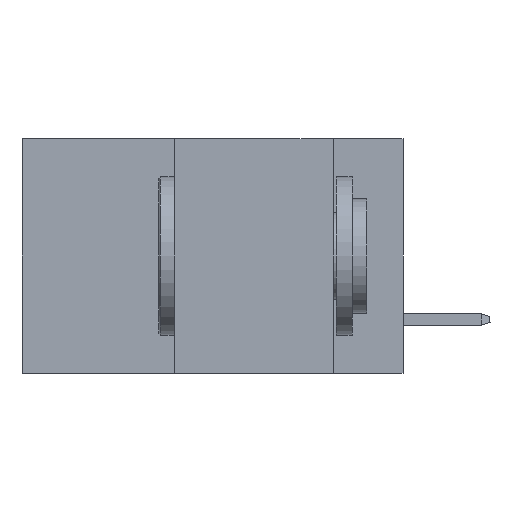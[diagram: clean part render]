
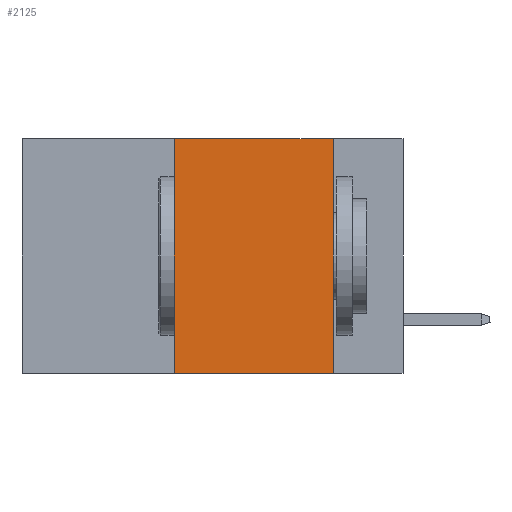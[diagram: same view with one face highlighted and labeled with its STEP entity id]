
A CAD part, left-side view. The second image highlights one B-rep face of the part: STEP entity #2125.
In plain terms, the highlighted planar face has unit normal (-1, 0, 0).
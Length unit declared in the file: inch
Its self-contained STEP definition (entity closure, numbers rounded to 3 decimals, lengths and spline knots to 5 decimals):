
#543 = VECTOR ( 'NONE', #2088, 39.37008 ) ;
#1757 = DIRECTION ( 'NONE',  ( 0., 0., -1. ) ) ;
#2088 = DIRECTION ( 'NONE',  ( 0., -1., 0. ) ) ;
#2125 = ADVANCED_FACE ( 'NONE', ( #6250 ), #36952, .F. ) ;
#2685 = CARTESIAN_POINT ( 'NONE',  ( 0., 0.36, -0.37 ) ) ;
#3008 = ORIENTED_EDGE ( 'NONE', *, *, #6449, .F. ) ;
#3105 = VECTOR ( 'NONE', #20566, 39.37008 ) ;
#5437 = LINE ( 'NONE', #5630, #23436 ) ;
#5608 = ORIENTED_EDGE ( 'NONE', *, *, #9338, .F. ) ;
#5630 = CARTESIAN_POINT ( 'NONE',  ( 0., 0.36, 0. ) ) ;
#6250 = FACE_OUTER_BOUND ( 'NONE', #6579, .T. ) ;
#6449 = EDGE_CURVE ( 'NONE', #37392, #36360, #20601, .T. ) ;
#6579 = EDGE_LOOP ( 'NONE', ( #3008, #27187, #5608, #22698 ) ) ;
#8728 = CARTESIAN_POINT ( 'NONE',  ( 0., 0.6, -0.37 ) ) ;
#9338 = EDGE_CURVE ( 'NONE', #34273, #24381, #5437, .T. ) ;
#12733 = DIRECTION ( 'NONE',  ( 0., 0., -1. ) ) ;
#13018 = AXIS2_PLACEMENT_3D ( 'NONE', #18644, #28104, #12733 ) ;
#14041 = VECTOR ( 'NONE', #1757, 39.37008 ) ;
#18644 = CARTESIAN_POINT ( 'NONE',  ( 0., 0.6, 0. ) ) ;
#20190 = CARTESIAN_POINT ( 'NONE',  ( 0., 0.11, 0. ) ) ;
#20566 = DIRECTION ( 'NONE',  ( 0., -1., 0. ) ) ;
#20601 = LINE ( 'NONE', #20190, #14041 ) ;
#20987 = LINE ( 'NONE', #23373, #3105 ) ;
#22698 = ORIENTED_EDGE ( 'NONE', *, *, #31850, .T. ) ;
#23373 = CARTESIAN_POINT ( 'NONE',  ( 0., 0.6, 0. ) ) ;
#23435 = CARTESIAN_POINT ( 'NONE',  ( 0., 0.11, -0.37 ) ) ;
#23436 = VECTOR ( 'NONE', #29901, 39.37008 ) ;
#24381 = VERTEX_POINT ( 'NONE', #31854 ) ;
#27187 = ORIENTED_EDGE ( 'NONE', *, *, #35748, .F. ) ;
#28104 = DIRECTION ( 'NONE',  ( 1., 0., 0. ) ) ;
#29901 = DIRECTION ( 'NONE',  ( 0., 0., 1. ) ) ;
#30391 = CARTESIAN_POINT ( 'NONE',  ( 0., 0.11, 0. ) ) ;
#31850 = EDGE_CURVE ( 'NONE', #34273, #36360, #36402, .T. ) ;
#31854 = CARTESIAN_POINT ( 'NONE',  ( 0., 0.36, 0. ) ) ;
#34273 = VERTEX_POINT ( 'NONE', #2685 ) ;
#35748 = EDGE_CURVE ( 'NONE', #24381, #37392, #20987, .T. ) ;
#36360 = VERTEX_POINT ( 'NONE', #23435 ) ;
#36402 = LINE ( 'NONE', #8728, #543 ) ;
#36952 = PLANE ( 'NONE',  #13018 ) ;
#37392 = VERTEX_POINT ( 'NONE', #30391 ) ;
